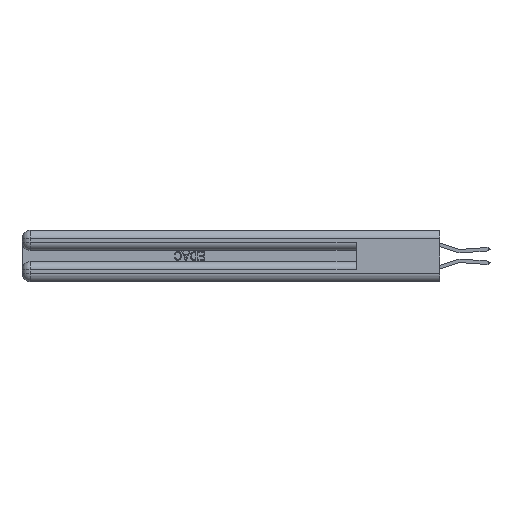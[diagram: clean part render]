
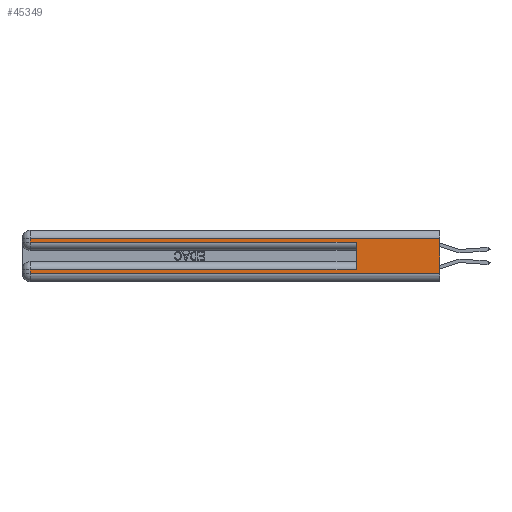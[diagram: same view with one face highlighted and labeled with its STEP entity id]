
A CAD part, left-side view. The second image highlights one B-rep face of the part: STEP entity #45349.
In plain terms, the highlighted planar face has unit normal (-1, 0, 0).
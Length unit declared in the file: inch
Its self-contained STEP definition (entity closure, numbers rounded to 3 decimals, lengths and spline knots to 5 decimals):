
#483 = ORIENTED_EDGE ( 'NONE', *, *, #13594, .T. ) ;
#1936 = CARTESIAN_POINT ( 'NONE',  ( 0., 0., 0.37 ) ) ;
#1964 = CARTESIAN_POINT ( 'NONE',  ( 0., 2.94, 0.31 ) ) ;
#3461 = DIRECTION ( 'NONE',  ( 0., 0., -1. ) ) ;
#3501 = VERTEX_POINT ( 'NONE', #6350 ) ;
#4037 = EDGE_CURVE ( 'NONE', #22875, #39454, #16213, .T. ) ;
#4172 = VERTEX_POINT ( 'NONE', #29745 ) ;
#5181 = CARTESIAN_POINT ( 'NONE',  ( 0., 2.94, 0.285 ) ) ;
#6121 = DIRECTION ( 'NONE',  ( 0., -1., 0. ) ) ;
#6350 = CARTESIAN_POINT ( 'NONE',  ( 0., 2.94, 0.085 ) ) ;
#7841 = ORIENTED_EDGE ( 'NONE', *, *, #4037, .F. ) ;
#8003 = DIRECTION ( 'NONE',  ( 0., 0., -1. ) ) ;
#8678 = DIRECTION ( 'NONE',  ( 1., 0., 0. ) ) ;
#8697 = EDGE_CURVE ( 'NONE', #10583, #28404, #23494, .T. ) ;
#8699 = VERTEX_POINT ( 'NONE', #1964 ) ;
#9953 = CARTESIAN_POINT ( 'NONE',  ( 0., 0., 0.06 ) ) ;
#10583 = VERTEX_POINT ( 'NONE', #23307 ) ;
#10847 = DIRECTION ( 'NONE',  ( 0., 0., -1. ) ) ;
#11281 = LINE ( 'NONE', #12311, #18364 ) ;
#12311 = CARTESIAN_POINT ( 'NONE',  ( 0., 0., 0.31 ) ) ;
#13111 = ORIENTED_EDGE ( 'NONE', *, *, #47962, .T. ) ;
#13392 = VECTOR ( 'NONE', #6121, 39.37008 ) ;
#13494 = VECTOR ( 'NONE', #3461, 39.37008 ) ;
#13594 = EDGE_CURVE ( 'NONE', #8699, #43386, #40289, .T. ) ;
#13909 = ORIENTED_EDGE ( 'NONE', *, *, #8697, .T. ) ;
#14349 = CARTESIAN_POINT ( 'NONE',  ( 0., 2.94, 0.37 ) ) ;
#14982 = VECTOR ( 'NONE', #25690, 39.37008 ) ;
#15453 = DIRECTION ( 'NONE',  ( 0., 1., 0. ) ) ;
#15530 = CARTESIAN_POINT ( 'NONE',  ( 0., 0.6, 0.085 ) ) ;
#16213 = LINE ( 'NONE', #29974, #14982 ) ;
#16764 = ORIENTED_EDGE ( 'NONE', *, *, #26851, .T. ) ;
#17219 = DIRECTION ( 'NONE',  ( 0., 1., 0. ) ) ;
#17289 = LINE ( 'NONE', #18953, #26150 ) ;
#17416 = ORIENTED_EDGE ( 'NONE', *, *, #29884, .T. ) ;
#18364 = VECTOR ( 'NONE', #15453, 39.37008 ) ;
#18953 = CARTESIAN_POINT ( 'NONE',  ( 0., 0., 0.285 ) ) ;
#19322 = LINE ( 'NONE', #1936, #26996 ) ;
#22779 = DIRECTION ( 'NONE',  ( 0., -1., 0. ) ) ;
#22875 = VERTEX_POINT ( 'NONE', #15530 ) ;
#23307 = CARTESIAN_POINT ( 'NONE',  ( 0., 2.94, 0.06 ) ) ;
#23494 = LINE ( 'NONE', #32603, #13392 ) ;
#23584 = AXIS2_PLACEMENT_3D ( 'NONE', #46139, #8678, #8003 ) ;
#24769 = VECTOR ( 'NONE', #17219, 39.37008 ) ;
#25002 = DIRECTION ( 'NONE',  ( 0., 0., -1. ) ) ;
#25690 = DIRECTION ( 'NONE',  ( 0., 0., 1. ) ) ;
#26043 = CARTESIAN_POINT ( 'NONE',  ( 0., 2.94, 0.37 ) ) ;
#26150 = VECTOR ( 'NONE', #22779, 39.37008 ) ;
#26851 = EDGE_CURVE ( 'NONE', #3501, #10583, #46478, .T. ) ;
#26996 = VECTOR ( 'NONE', #25002, 39.37008 ) ;
#28404 = VERTEX_POINT ( 'NONE', #9953 ) ;
#29745 = CARTESIAN_POINT ( 'NONE',  ( 0., 0., 0.31 ) ) ;
#29884 = EDGE_CURVE ( 'NONE', #43386, #39454, #17289, .T. ) ;
#29974 = CARTESIAN_POINT ( 'NONE',  ( 0., 0.6, 0.145 ) ) ;
#30072 = ORIENTED_EDGE ( 'NONE', *, *, #42803, .T. ) ;
#31272 = PLANE ( 'NONE',  #23584 ) ;
#32603 = CARTESIAN_POINT ( 'NONE',  ( 0., 0., 0.06 ) ) ;
#37029 = EDGE_CURVE ( 'NONE', #4172, #28404, #19322, .T. ) ;
#38552 = FACE_OUTER_BOUND ( 'NONE', #39617, .T. ) ;
#39454 = VERTEX_POINT ( 'NONE', #47693 ) ;
#39617 = EDGE_LOOP ( 'NONE', ( #39895, #13111, #483, #17416, #7841, #30072, #16764, #13909 ) ) ;
#39710 = CARTESIAN_POINT ( 'NONE',  ( 0., 0., 0.085 ) ) ;
#39895 = ORIENTED_EDGE ( 'NONE', *, *, #37029, .F. ) ;
#40289 = LINE ( 'NONE', #14349, #42705 ) ;
#42705 = VECTOR ( 'NONE', #10847, 39.37008 ) ;
#42803 = EDGE_CURVE ( 'NONE', #22875, #3501, #45866, .T. ) ;
#43386 = VERTEX_POINT ( 'NONE', #5181 ) ;
#45349 = ADVANCED_FACE ( 'NONE', ( #38552 ), #31272, .F. ) ;
#45866 = LINE ( 'NONE', #39710, #24769 ) ;
#46139 = CARTESIAN_POINT ( 'NONE',  ( 0., 0., 0.37 ) ) ;
#46478 = LINE ( 'NONE', #26043, #13494 ) ;
#47693 = CARTESIAN_POINT ( 'NONE',  ( 0., 0.6, 0.285 ) ) ;
#47962 = EDGE_CURVE ( 'NONE', #4172, #8699, #11281, .T. ) ;
